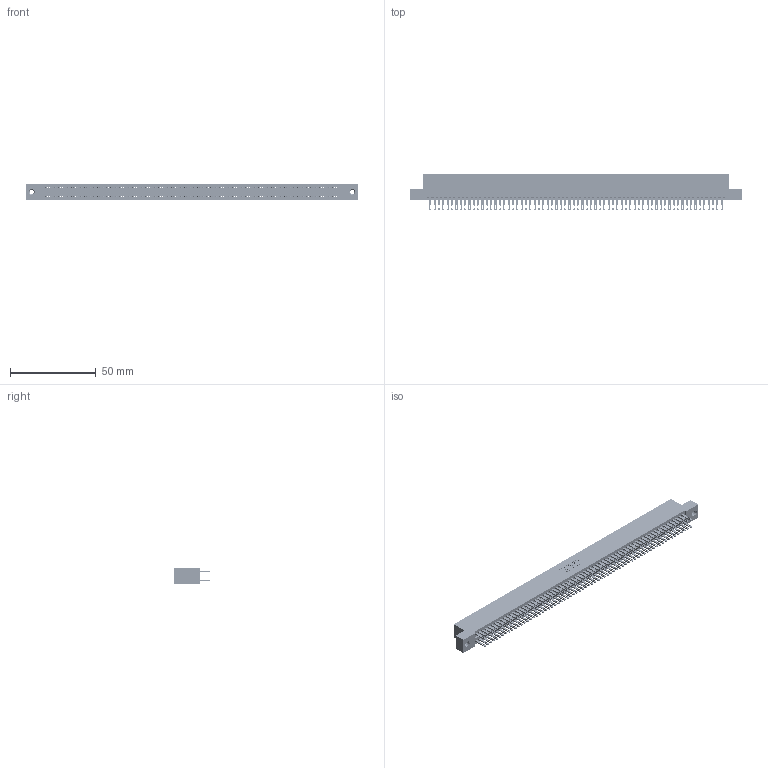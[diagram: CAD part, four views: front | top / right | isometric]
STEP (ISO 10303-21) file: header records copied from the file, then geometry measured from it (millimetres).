
FILE_DESCRIPTION (( 'STEP AP203' ), '1' );
FILE_NAME ('895-136-500-207.STEP', '2020-10-13T18:20:43', ( '' ), ( '' ), 'SwSTEP 2.0', 'SolidWorks 2020', '' );
FILE_SCHEMA (( 'CONFIG_CONTROL_DESIGN' ));
Length unit declared in the file: inch
Products named in the file (4): 345-292-001_345-293-100; 345-250-001_345-250-005-103; 895-136-500-207; 845 Part_Flush Mounting Lugs - 0.156 Dia-TI
Assembly tree (139 placements, depth 2):
  895-136-500-207
    845 Part_Flush Mounting Lugs - 0.156 Dia-TI
    345-292-001_345-293-100  x136
    345-250-001_345-250-005-103  x2
Bounding box: 193.93 x 21.51 x 9.4 mm (x, y, z)
Volume: 19481.9 mm3; surface area: 30716.1 mm2
Topology: 139 solids, 139 shells, 6442 faces, 19653 edges, 13094 vertices
Faces by surface type: plane 3784, cylinder 2642, cone 12, torus 4
Entity records: 50970 total; most frequent: CARTESIAN_POINT 8499, ORIENTED_EDGE 8426, DIRECTION 7491, EDGE_CURVE 4213, LINE 3785, VECTOR 3785, VERTEX_POINT 2804, AXIS2_PLACEMENT_3D 1853
